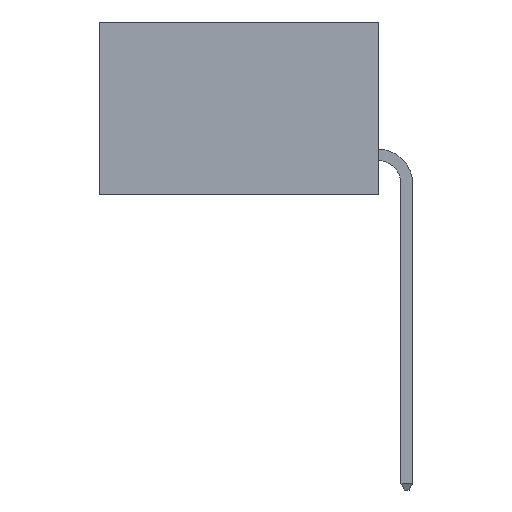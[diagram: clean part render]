
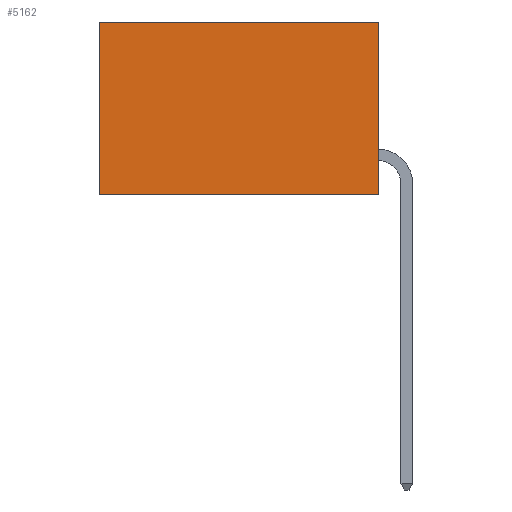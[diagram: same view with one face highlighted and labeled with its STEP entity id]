
A CAD part, left-side view. The second image highlights one B-rep face of the part: STEP entity #5162.
In plain terms, the highlighted planar face has unit normal (-1, 0, 0).
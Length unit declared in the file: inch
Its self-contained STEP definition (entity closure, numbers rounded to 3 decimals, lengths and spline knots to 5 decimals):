
#367 = VECTOR ( 'NONE', #8223, 39.37008 ) ;
#378 = CARTESIAN_POINT ( 'NONE',  ( 0.298, 0.6, 0. ) ) ;
#1163 = VECTOR ( 'NONE', #6904, 39.37008 ) ;
#1179 = DIRECTION ( 'NONE',  ( 0., 1., 0. ) ) ;
#2464 = DIRECTION ( 'NONE',  ( 0., 0., -1. ) ) ;
#3036 = CARTESIAN_POINT ( 'NONE',  ( 0.298, 0.6, 0. ) ) ;
#3377 = VERTEX_POINT ( 'NONE', #7541 ) ;
#3516 = CARTESIAN_POINT ( 'NONE',  ( 0.298, 0., 0. ) ) ;
#4328 = LINE ( 'NONE', #5866, #1163 ) ;
#4488 = VERTEX_POINT ( 'NONE', #6470 ) ;
#4609 = LINE ( 'NONE', #12258, #7356 ) ;
#4808 = ORIENTED_EDGE ( 'NONE', *, *, #9770, .T. ) ;
#4820 = EDGE_CURVE ( 'NONE', #3377, #5135, #4609, .T. ) ;
#5135 = VERTEX_POINT ( 'NONE', #378 ) ;
#5162 = ADVANCED_FACE ( 'NONE', ( #8936 ), #5956, .F. ) ;
#5546 = ORIENTED_EDGE ( 'NONE', *, *, #4820, .T. ) ;
#5643 = VERTEX_POINT ( 'NONE', #6106 ) ;
#5866 = CARTESIAN_POINT ( 'NONE',  ( 0.298, 0., 0. ) ) ;
#5956 = PLANE ( 'NONE',  #9119 ) ;
#6106 = CARTESIAN_POINT ( 'NONE',  ( 0.298, 0.6, -0.37 ) ) ;
#6470 = CARTESIAN_POINT ( 'NONE',  ( 0.298, 0., -0.37 ) ) ;
#6904 = DIRECTION ( 'NONE',  ( 0., 0., -1. ) ) ;
#7356 = VECTOR ( 'NONE', #1179, 39.37008 ) ;
#7541 = CARTESIAN_POINT ( 'NONE',  ( 0.298, 0., 0. ) ) ;
#7719 = VECTOR ( 'NONE', #11963, 39.37008 ) ;
#8116 = CARTESIAN_POINT ( 'NONE',  ( 0.298, 0., -0.37 ) ) ;
#8223 = DIRECTION ( 'NONE',  ( 0., 0., -1. ) ) ;
#8591 = EDGE_CURVE ( 'NONE', #3377, #4488, #4328, .T. ) ;
#8936 = FACE_OUTER_BOUND ( 'NONE', #12257, .T. ) ;
#9038 = DIRECTION ( 'NONE',  ( 1., 0., 0. ) ) ;
#9119 = AXIS2_PLACEMENT_3D ( 'NONE', #3516, #9038, #2464 ) ;
#9770 = EDGE_CURVE ( 'NONE', #5135, #5643, #11348, .T. ) ;
#10278 = ORIENTED_EDGE ( 'NONE', *, *, #12555, .F. ) ;
#10351 = LINE ( 'NONE', #8116, #7719 ) ;
#10470 = ORIENTED_EDGE ( 'NONE', *, *, #8591, .F. ) ;
#11348 = LINE ( 'NONE', #3036, #367 ) ;
#11963 = DIRECTION ( 'NONE',  ( 0., 1., 0. ) ) ;
#12257 = EDGE_LOOP ( 'NONE', ( #4808, #10278, #10470, #5546 ) ) ;
#12258 = CARTESIAN_POINT ( 'NONE',  ( 0.298, 0., 0. ) ) ;
#12555 = EDGE_CURVE ( 'NONE', #4488, #5643, #10351, .T. ) ;
